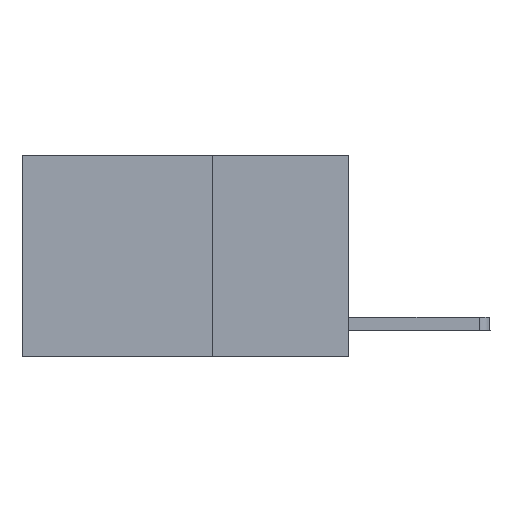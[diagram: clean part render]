
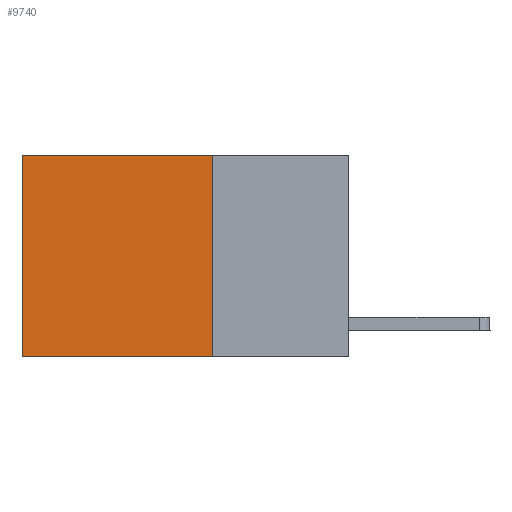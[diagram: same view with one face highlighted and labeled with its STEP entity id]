
A CAD part, left-side view. The second image highlights one B-rep face of the part: STEP entity #9740.
In plain terms, the highlighted planar face has unit normal (-1, 0, 0).
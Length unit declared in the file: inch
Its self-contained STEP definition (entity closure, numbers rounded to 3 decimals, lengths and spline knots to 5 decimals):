
#39 = CARTESIAN_POINT ( 'NONE',  ( 0.2625, 0.25, -0.37 ) ) ;
#233 = CARTESIAN_POINT ( 'NONE',  ( 0.2625, 0.25, 0. ) ) ;
#475 = CARTESIAN_POINT ( 'NONE',  ( 0.2625, 0.25, 0. ) ) ;
#1100 = ORIENTED_EDGE ( 'NONE', *, *, #4036, .T. ) ;
#2199 = DIRECTION ( 'NONE',  ( 0., 0., -1. ) ) ;
#2725 = DIRECTION ( 'NONE',  ( 0., 1., 0. ) ) ;
#2822 = CARTESIAN_POINT ( 'NONE',  ( 0.2625, 0.25, -0.37 ) ) ;
#2847 = EDGE_CURVE ( 'NONE', #4657, #2905, #9723, .T. ) ;
#2878 = LINE ( 'NONE', #2822, #2929 ) ;
#2891 = LINE ( 'NONE', #8965, #4683 ) ;
#2905 = VERTEX_POINT ( 'NONE', #8294 ) ;
#2929 = VECTOR ( 'NONE', #8952, 39.37008 ) ;
#3324 = DIRECTION ( 'NONE',  ( 0., 0., -1. ) ) ;
#3443 = CARTESIAN_POINT ( 'NONE',  ( 0.2625, 0.25, 0. ) ) ;
#3721 = EDGE_CURVE ( 'NONE', #8370, #8205, #2891, .T. ) ;
#4036 = EDGE_CURVE ( 'NONE', #8370, #4657, #9690, .T. ) ;
#4049 = EDGE_CURVE ( 'NONE', #8205, #2905, #2878, .T. ) ;
#4071 = PLANE ( 'NONE',  #8327 ) ;
#4657 = VERTEX_POINT ( 'NONE', #7507 ) ;
#4683 = VECTOR ( 'NONE', #6592, 39.37008 ) ;
#4778 = EDGE_LOOP ( 'NONE', ( #8532, #5765, #5503, #1100 ) ) ;
#5503 = ORIENTED_EDGE ( 'NONE', *, *, #3721, .F. ) ;
#5535 = DIRECTION ( 'NONE',  ( 1., 0., 0. ) ) ;
#5765 = ORIENTED_EDGE ( 'NONE', *, *, #4049, .F. ) ;
#5928 = VECTOR ( 'NONE', #2199, 39.37008 ) ;
#6592 = DIRECTION ( 'NONE',  ( 0., 0., -1. ) ) ;
#6760 = CARTESIAN_POINT ( 'NONE',  ( 0.2625, 0.6, 0. ) ) ;
#7507 = CARTESIAN_POINT ( 'NONE',  ( 0.2625, 0.6, 0. ) ) ;
#8205 = VERTEX_POINT ( 'NONE', #39 ) ;
#8294 = CARTESIAN_POINT ( 'NONE',  ( 0.2625, 0.6, -0.37 ) ) ;
#8327 = AXIS2_PLACEMENT_3D ( 'NONE', #233, #5535, #3324 ) ;
#8370 = VERTEX_POINT ( 'NONE', #475 ) ;
#8532 = ORIENTED_EDGE ( 'NONE', *, *, #2847, .T. ) ;
#8952 = DIRECTION ( 'NONE',  ( 0., 1., 0. ) ) ;
#8965 = CARTESIAN_POINT ( 'NONE',  ( 0.2625, 0.25, 0. ) ) ;
#9369 = FACE_OUTER_BOUND ( 'NONE', #4778, .T. ) ;
#9690 = LINE ( 'NONE', #3443, #9692 ) ;
#9692 = VECTOR ( 'NONE', #2725, 39.37008 ) ;
#9723 = LINE ( 'NONE', #6760, #5928 ) ;
#9740 = ADVANCED_FACE ( 'NONE', ( #9369 ), #4071, .F. ) ;
